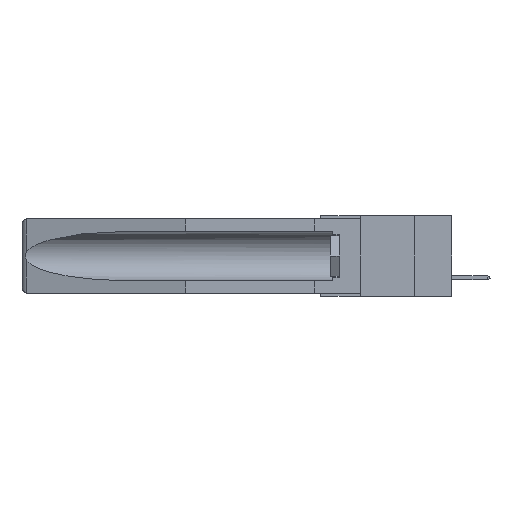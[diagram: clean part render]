
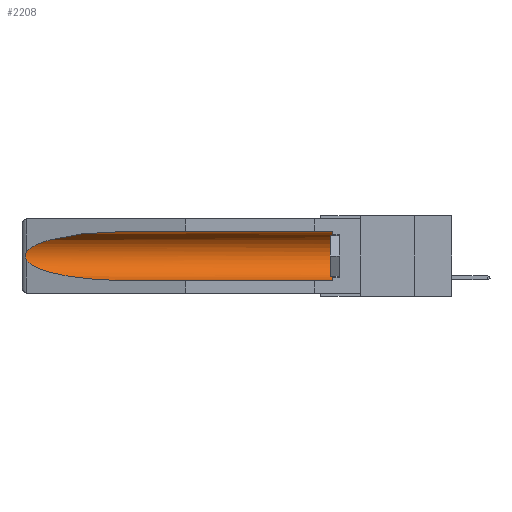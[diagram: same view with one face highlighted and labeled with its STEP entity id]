
A CAD part, left-side view. The second image highlights one B-rep face of the part: STEP entity #2208.
In plain terms, the highlighted cylindrical face has radius 2.857 mm (diameter 5.715 mm), a partial arc.
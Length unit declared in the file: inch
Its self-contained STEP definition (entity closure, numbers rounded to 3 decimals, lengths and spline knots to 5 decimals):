
#216 = LINE ( 'NONE', #5118, #12488 ) ;
#396 = CARTESIAN_POINT ( 'NONE',  ( 0.26537, 1.52718, -0.19328 ) ) ;
#1086 = DIRECTION ( 'NONE',  ( 0., 0., 1. ) ) ;
#1175 = EDGE_CURVE ( 'NONE', #10551, #13605, #18682, .T. ) ;
#1902 = DIRECTION ( 'NONE',  ( 0., 1., 0. ) ) ;
#2208 = ADVANCED_FACE ( 'NONE', ( #8557 ), #17152, .F. ) ;
#2644 = B_SPLINE_CURVE_WITH_KNOTS ( 'NONE', 3,
 ( #12309, #16868, #13606, #4206, #4482, #16993, #15354, #16806, #10665, #4417 ),
 .UNSPECIFIED., .F., .F.,
 ( 4, 2, 2, 2, 4 ),
 ( 0., 0.00029, 0.00058, 0.00087, 0.00117 ),
 .UNSPECIFIED. ) ;
#2956 = LINE ( 'NONE', #17572, #19208 ) ;
#3219 = DIRECTION ( 'NONE',  ( 0., 0., 1. ) ) ;
#3272 = CARTESIAN_POINT ( 'NONE',  ( 0.26537, 1.52718, -0.14972 ) ) ;
#3342 = CARTESIAN_POINT ( 'NONE',  ( 0.21114, 1.30732, -0.059 ) ) ;
#3381 = EDGE_CURVE ( 'NONE', #10551, #7574, #2956, .T. ) ;
#4206 = CARTESIAN_POINT ( 'NONE',  ( 0.2673, 1.5327, -0.16383 ) ) ;
#4224 = EDGE_CURVE ( 'NONE', #13605, #14285, #216, .T. ) ;
#4417 = CARTESIAN_POINT ( 'NONE',  ( 0.26537, 1.52718, -0.19328 ) ) ;
#4482 = CARTESIAN_POINT ( 'NONE',  ( 0.2675, 1.53308, -0.16763 ) ) ;
#5118 = CARTESIAN_POINT ( 'NONE',  ( 0.155, -0.30754, -0.059 ) ) ;
#5741 = CARTESIAN_POINT ( 'NONE',  ( 0.25451, 1.48313, -0.24835 ) ) ;
#5909 = EDGE_CURVE ( 'NONE', #6795, #6636, #2644, .T. ) ;
#6636 = VERTEX_POINT ( 'NONE', #396 ) ;
#6795 = VERTEX_POINT ( 'NONE', #3272 ) ;
#7165 =( BOUNDED_CURVE ( )  B_SPLINE_CURVE ( 3, ( #15171, #5741, #8872, #13302 ),
 .UNSPECIFIED., .F., .F. ) 
 B_SPLINE_CURVE_WITH_KNOTS ( ( 4, 4 ),
 ( 0.1948, 1.5708 ),
 .UNSPECIFIED. ) 
 CURVE ( )  GEOMETRIC_REPRESENTATION_ITEM ( )  RATIONAL_B_SPLINE_CURVE ( ( 1., 0.848, 0.848, 1. ) ) 
 REPRESENTATION_ITEM ( '' )  );
#7410 = CARTESIAN_POINT ( 'NONE',  ( 0.155, 0.126, -0.1715 ) ) ;
#7415 = EDGE_CURVE ( 'NONE', #14285, #6795, #7421, .T. ) ;
#7421 =( BOUNDED_CURVE ( )  B_SPLINE_CURVE ( 3, ( #11446, #3342, #16693, #8812 ),
 .UNSPECIFIED., .F., .F. ) 
 B_SPLINE_CURVE_WITH_KNOTS ( ( 4, 4 ),
 ( 4.71239, 6.08839 ),
 .UNSPECIFIED. ) 
 CURVE ( )  GEOMETRIC_REPRESENTATION_ITEM ( )  RATIONAL_B_SPLINE_CURVE ( ( 1., 0.848, 0.848, 1. ) ) 
 REPRESENTATION_ITEM ( '' )  );
#7574 = VERTEX_POINT ( 'NONE', #12109 ) ;
#8557 = FACE_OUTER_BOUND ( 'NONE', #16117, .T. ) ;
#8812 = CARTESIAN_POINT ( 'NONE',  ( 0.26537, 1.52718, -0.14972 ) ) ;
#8872 = CARTESIAN_POINT ( 'NONE',  ( 0.21114, 1.30732, -0.284 ) ) ;
#9249 = ORIENTED_EDGE ( 'NONE', *, *, #17164, .T. ) ;
#10023 = ORIENTED_EDGE ( 'NONE', *, *, #5909, .T. ) ;
#10490 = DIRECTION ( 'NONE',  ( 0., -1., 0. ) ) ;
#10551 = VERTEX_POINT ( 'NONE', #11131 ) ;
#10665 = CARTESIAN_POINT ( 'NONE',  ( 0.26597, 1.5296, -0.19026 ) ) ;
#11131 = CARTESIAN_POINT ( 'NONE',  ( 0.155, 0.126, -0.284 ) ) ;
#11446 = CARTESIAN_POINT ( 'NONE',  ( 0.155, 1.07973, -0.059 ) ) ;
#12109 = CARTESIAN_POINT ( 'NONE',  ( 0.155, 1.07973, -0.284 ) ) ;
#12309 = CARTESIAN_POINT ( 'NONE',  ( 0.26537, 1.52718, -0.14972 ) ) ;
#12488 = VECTOR ( 'NONE', #17690, 39.37008 ) ;
#12695 = DIRECTION ( 'NONE',  ( 0., 1., 0. ) ) ;
#13263 = ORIENTED_EDGE ( 'NONE', *, *, #3381, .F. ) ;
#13302 = CARTESIAN_POINT ( 'NONE',  ( 0.155, 1.07973, -0.284 ) ) ;
#13605 = VERTEX_POINT ( 'NONE', #18560 ) ;
#13606 = CARTESIAN_POINT ( 'NONE',  ( 0.26654, 1.53092, -0.15636 ) ) ;
#14250 = AXIS2_PLACEMENT_3D ( 'NONE', #7410, #10490, #1086 ) ;
#14285 = VERTEX_POINT ( 'NONE', #18507 ) ;
#15171 = CARTESIAN_POINT ( 'NONE',  ( 0.26537, 1.52718, -0.19328 ) ) ;
#15214 = ORIENTED_EDGE ( 'NONE', *, *, #4224, .T. ) ;
#15354 = CARTESIAN_POINT ( 'NONE',  ( 0.2673, 1.53269, -0.17917 ) ) ;
#15750 = ORIENTED_EDGE ( 'NONE', *, *, #1175, .T. ) ;
#16117 = EDGE_LOOP ( 'NONE', ( #19389, #10023, #9249, #13263, #15750, #15214 ) ) ;
#16693 = CARTESIAN_POINT ( 'NONE',  ( 0.25451, 1.48313, -0.09465 ) ) ;
#16806 = CARTESIAN_POINT ( 'NONE',  ( 0.26655, 1.53094, -0.18657 ) ) ;
#16868 = CARTESIAN_POINT ( 'NONE',  ( 0.26597, 1.52961, -0.15275 ) ) ;
#16993 = CARTESIAN_POINT ( 'NONE',  ( 0.2675, 1.53308, -0.17534 ) ) ;
#17152 = CYLINDRICAL_SURFACE ( 'NONE', #18613, 0.1125 ) ;
#17164 = EDGE_CURVE ( 'NONE', #6636, #7574, #7165, .T. ) ;
#17572 = CARTESIAN_POINT ( 'NONE',  ( 0.155, -0.30754, -0.284 ) ) ;
#17690 = DIRECTION ( 'NONE',  ( 0., 1., 0. ) ) ;
#18507 = CARTESIAN_POINT ( 'NONE',  ( 0.155, 1.07973, -0.059 ) ) ;
#18560 = CARTESIAN_POINT ( 'NONE',  ( 0.155, 0.126, -0.059 ) ) ;
#18613 = AXIS2_PLACEMENT_3D ( 'NONE', #19037, #12695, #3219 ) ;
#18682 = CIRCLE ( 'NONE', #14250, 0.1125 ) ;
#19037 = CARTESIAN_POINT ( 'NONE',  ( 0.155, -0.30754, -0.1715 ) ) ;
#19208 = VECTOR ( 'NONE', #1902, 39.37008 ) ;
#19389 = ORIENTED_EDGE ( 'NONE', *, *, #7415, .T. ) ;
